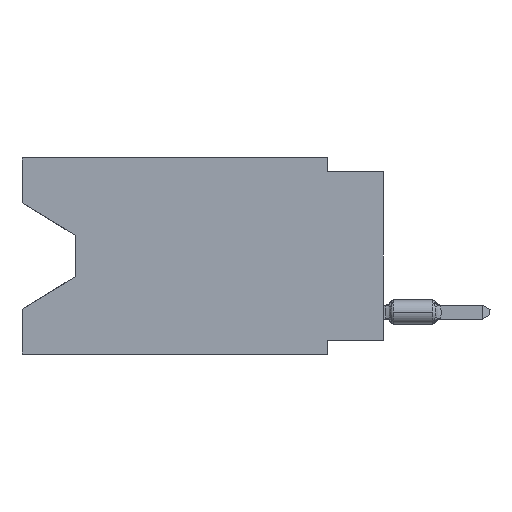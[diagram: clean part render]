
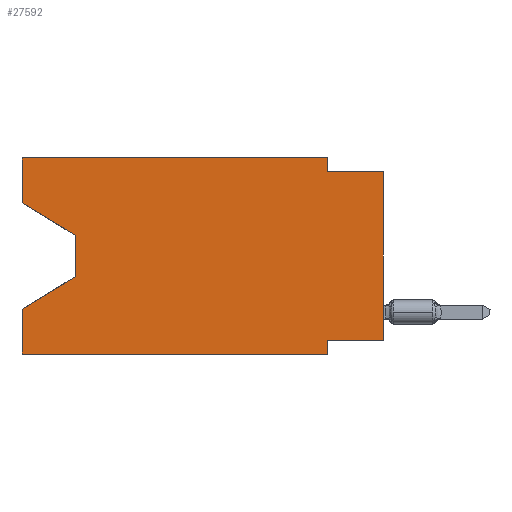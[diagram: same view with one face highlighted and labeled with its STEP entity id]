
A CAD part, left-side view. The second image highlights one B-rep face of the part: STEP entity #27592.
In plain terms, the highlighted planar face has unit normal (-1, 0, 0).
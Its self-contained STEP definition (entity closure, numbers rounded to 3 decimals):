
#622 = CARTESIAN_POINT ( 'NONE',  ( 0., 0., -0.635 ) ) ;
#755 = CARTESIAN_POINT ( 'NONE',  ( 0., 13.97, -5.385 ) ) ;
#809 = CARTESIAN_POINT ( 'NONE',  ( 0., 16.383, 0. ) ) ;
#816 = VERTEX_POINT ( 'NONE', #22288 ) ;
#918 = LINE ( 'NONE', #10472, #41691 ) ;
#1017 = LINE ( 'NONE', #809, #33258 ) ;
#1593 = EDGE_CURVE ( 'NONE', #2084, #25212, #18460, .T. ) ;
#1918 = LINE ( 'NONE', #15173, #9058 ) ;
#2084 = VERTEX_POINT ( 'NONE', #22099 ) ;
#2155 = DIRECTION ( 'NONE',  ( 0., 0., -1. ) ) ;
#2622 = VECTOR ( 'NONE', #9030, 1000. ) ;
#2650 = CARTESIAN_POINT ( 'NONE',  ( 0., 2.54, -8.255 ) ) ;
#2716 = ORIENTED_EDGE ( 'NONE', *, *, #1593, .T. ) ;
#3834 = ORIENTED_EDGE ( 'NONE', *, *, #30438, .F. ) ;
#4002 = ORIENTED_EDGE ( 'NONE', *, *, #9696, .F. ) ;
#4770 = FACE_OUTER_BOUND ( 'NONE', #36192, .T. ) ;
#4879 = EDGE_CURVE ( 'NONE', #32131, #25212, #13871, .T. ) ;
#5800 = ORIENTED_EDGE ( 'NONE', *, *, #36271, .F. ) ;
#7473 = CARTESIAN_POINT ( 'NONE',  ( 0., 16.383, 0. ) ) ;
#7502 = EDGE_CURVE ( 'NONE', #30109, #20195, #1017, .T. ) ;
#7622 = LINE ( 'NONE', #20873, #38607 ) ;
#9030 = DIRECTION ( 'NONE',  ( 0., -0.855, -0.519 ) ) ;
#9058 = VECTOR ( 'NONE', #2155, 1000. ) ;
#9392 = CARTESIAN_POINT ( 'NONE',  ( 0., 16.383, -2.038 ) ) ;
#9449 = LINE ( 'NONE', #28315, #2622 ) ;
#9696 = EDGE_CURVE ( 'NONE', #10730, #32131, #918, .T. ) ;
#9752 = ORIENTED_EDGE ( 'NONE', *, *, #34869, .F. ) ;
#10156 = LINE ( 'NONE', #23399, #22475 ) ;
#10456 = ORIENTED_EDGE ( 'NONE', *, *, #23526, .T. ) ;
#10472 = CARTESIAN_POINT ( 'NONE',  ( 0., 0., -8.255 ) ) ;
#10584 = DIRECTION ( 'NONE',  ( 0., 0., -1. ) ) ;
#10730 = VERTEX_POINT ( 'NONE', #33420 ) ;
#10825 = LINE ( 'NONE', #622, #11595 ) ;
#11595 = VECTOR ( 'NONE', #30344, 1000. ) ;
#11712 = CARTESIAN_POINT ( 'NONE',  ( 0., 16.383, 0. ) ) ;
#11882 = VERTEX_POINT ( 'NONE', #35667 ) ;
#12330 = VECTOR ( 'NONE', #25453, 1000. ) ;
#13308 = DIRECTION ( 'NONE',  ( 0., 1., 0. ) ) ;
#13608 = DIRECTION ( 'NONE',  ( 0., 0., 1. ) ) ;
#13871 = LINE ( 'NONE', #27103, #39844 ) ;
#14069 = CARTESIAN_POINT ( 'NONE',  ( 0., 2.54, -0.635 ) ) ;
#14495 = EDGE_CURVE ( 'NONE', #42435, #42713, #1918, .T. ) ;
#15173 = CARTESIAN_POINT ( 'NONE',  ( 0., 13.97, -3.505 ) ) ;
#16405 = DIRECTION ( 'NONE',  ( 0., 0.855, -0.519 ) ) ;
#16526 = EDGE_CURVE ( 'NONE', #11882, #20801, #23830, .T. ) ;
#17103 = ORIENTED_EDGE ( 'NONE', *, *, #16526, .F. ) ;
#17107 = CARTESIAN_POINT ( 'NONE',  ( 0., 2.54, 0. ) ) ;
#17602 = ORIENTED_EDGE ( 'NONE', *, *, #22254, .T. ) ;
#17827 = EDGE_CURVE ( 'NONE', #10730, #29988, #10156, .T. ) ;
#18027 = DIRECTION ( 'NONE',  ( 1., 0., 0. ) ) ;
#18460 = LINE ( 'NONE', #24964, #25199 ) ;
#20195 = VERTEX_POINT ( 'NONE', #7473 ) ;
#20801 = VERTEX_POINT ( 'NONE', #14069 ) ;
#20873 = CARTESIAN_POINT ( 'NONE',  ( 0., 16.383, 0. ) ) ;
#21118 = CARTESIAN_POINT ( 'NONE',  ( 0., 0., -0.635 ) ) ;
#21278 = DIRECTION ( 'NONE',  ( 0., -1., 0. ) ) ;
#22099 = CARTESIAN_POINT ( 'NONE',  ( 0., 16.383, -8.89 ) ) ;
#22254 = EDGE_CURVE ( 'NONE', #30109, #42435, #9449, .T. ) ;
#22288 = CARTESIAN_POINT ( 'NONE',  ( 0., 16.383, -6.852 ) ) ;
#22475 = VECTOR ( 'NONE', #36603, 1000. ) ;
#23399 = CARTESIAN_POINT ( 'NONE',  ( 0., 0., 0. ) ) ;
#23526 = EDGE_CURVE ( 'NONE', #42713, #816, #39372, .T. ) ;
#23830 = LINE ( 'NONE', #17107, #27192 ) ;
#24824 = ORIENTED_EDGE ( 'NONE', *, *, #4879, .F. ) ;
#24964 = CARTESIAN_POINT ( 'NONE',  ( 0., 16.383, -8.89 ) ) ;
#25199 = VECTOR ( 'NONE', #21278, 1000. ) ;
#25212 = VERTEX_POINT ( 'NONE', #35826 ) ;
#25383 = PLANE ( 'NONE',  #25994 ) ;
#25453 = DIRECTION ( 'NONE',  ( 0., 0., 1. ) ) ;
#25994 = AXIS2_PLACEMENT_3D ( 'NONE', #11712, #18027, #28182 ) ;
#26688 = ORIENTED_EDGE ( 'NONE', *, *, #7502, .F. ) ;
#27103 = CARTESIAN_POINT ( 'NONE',  ( 0., 2.54, -8.89 ) ) ;
#27192 = VECTOR ( 'NONE', #10584, 1000. ) ;
#27592 = ADVANCED_FACE ( 'NONE', ( #4770 ), #25383, .F. ) ;
#27618 = VECTOR ( 'NONE', #16405, 1000. ) ;
#28182 = DIRECTION ( 'NONE',  ( 0., 0., -1. ) ) ;
#28315 = CARTESIAN_POINT ( 'NONE',  ( 0., 16.383, -2.038 ) ) ;
#29988 = VERTEX_POINT ( 'NONE', #21118 ) ;
#30109 = VERTEX_POINT ( 'NONE', #9392 ) ;
#30344 = DIRECTION ( 'NONE',  ( 0., -1., 0. ) ) ;
#30438 = EDGE_CURVE ( 'NONE', #20195, #11882, #7622, .T. ) ;
#30829 = CARTESIAN_POINT ( 'NONE',  ( 0., 13.97, -3.505 ) ) ;
#31730 = LINE ( 'NONE', #32381, #12330 ) ;
#32131 = VERTEX_POINT ( 'NONE', #2650 ) ;
#32381 = CARTESIAN_POINT ( 'NONE',  ( 0., 16.383, 0. ) ) ;
#33258 = VECTOR ( 'NONE', #13608, 1000. ) ;
#33389 = DIRECTION ( 'NONE',  ( 0., 0., -1. ) ) ;
#33420 = CARTESIAN_POINT ( 'NONE',  ( 0., 0., -8.255 ) ) ;
#33576 = ORIENTED_EDGE ( 'NONE', *, *, #17827, .T. ) ;
#34674 = ORIENTED_EDGE ( 'NONE', *, *, #14495, .T. ) ;
#34869 = EDGE_CURVE ( 'NONE', #2084, #816, #31730, .T. ) ;
#35086 = DIRECTION ( 'NONE',  ( 0., -1., 0. ) ) ;
#35667 = CARTESIAN_POINT ( 'NONE',  ( 0., 2.54, 0. ) ) ;
#35826 = CARTESIAN_POINT ( 'NONE',  ( 0., 2.54, -8.89 ) ) ;
#36192 = EDGE_LOOP ( 'NONE', ( #17602, #34674, #10456, #9752, #2716, #24824, #4002, #33576, #5800, #17103, #3834, #26688 ) ) ;
#36271 = EDGE_CURVE ( 'NONE', #20801, #29988, #10825, .T. ) ;
#36603 = DIRECTION ( 'NONE',  ( 0., 0., 1. ) ) ;
#38607 = VECTOR ( 'NONE', #35086, 1000. ) ;
#39251 = CARTESIAN_POINT ( 'NONE',  ( 0., 13.97, -5.385 ) ) ;
#39372 = LINE ( 'NONE', #755, #27618 ) ;
#39844 = VECTOR ( 'NONE', #33389, 1000. ) ;
#41691 = VECTOR ( 'NONE', #13308, 1000. ) ;
#42435 = VERTEX_POINT ( 'NONE', #30829 ) ;
#42713 = VERTEX_POINT ( 'NONE', #39251 ) ;
